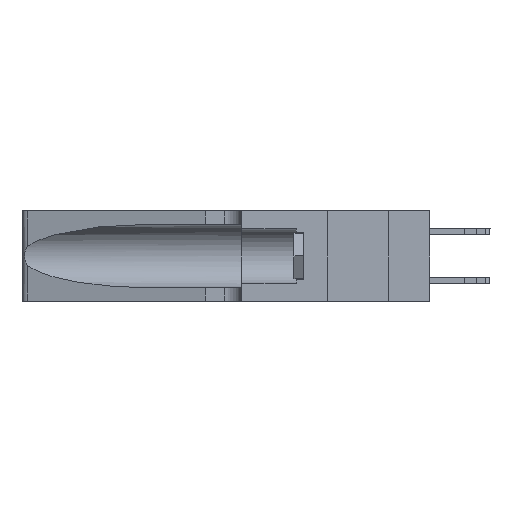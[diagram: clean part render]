
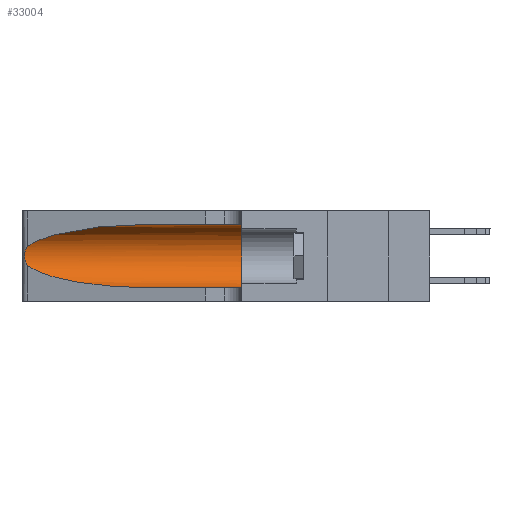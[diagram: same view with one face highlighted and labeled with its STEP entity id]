
A CAD part, left-side view. The second image highlights one B-rep face of the part: STEP entity #33004.
In plain terms, the highlighted cylindrical face has radius 3.308 mm (diameter 6.617 mm), a partial arc.
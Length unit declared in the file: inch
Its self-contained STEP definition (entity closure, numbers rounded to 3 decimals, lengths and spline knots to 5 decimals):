
#201 = CARTESIAN_POINT ( 'NONE',  ( 0.1305, 0.72297, 0.31525 ) ) ;
#750 = VERTEX_POINT ( 'NONE', #201 ) ;
#987 = VERTEX_POINT ( 'NONE', #16166 ) ;
#3765 = ORIENTED_EDGE ( 'NONE', *, *, #8868, .F. ) ;
#3880 = CARTESIAN_POINT ( 'NONE',  ( 0.2373, 1.15595, 0.08982 ) ) ;
#4283 = CARTESIAN_POINT ( 'NONE',  ( 0.1305, 0.72297, 0.05475 ) ) ;
#4322 = EDGE_CURVE ( 'NONE', #750, #6726, #26907, .T. ) ;
#4365 = CARTESIAN_POINT ( 'NONE',  ( 0.1305, 1.61858, 0.31525 ) ) ;
#5278 = ORIENTED_EDGE ( 'NONE', *, *, #11281, .T. ) ;
#5310 = CARTESIAN_POINT ( 'NONE',  ( 0.25856, 1.23593, 0.16098 ) ) ;
#6726 = VERTEX_POINT ( 'NONE', #12524 ) ;
#6749 = EDGE_CURVE ( 'NONE', #18286, #987, #23998, .T. ) ;
#8090 = CARTESIAN_POINT ( 'NONE',  ( 0.1305, 0.72297, 0.31525 ) ) ;
#8315 = VECTOR ( 'NONE', #16398, 39.37008 ) ;
#8562 = CARTESIAN_POINT ( 'NONE',  ( 0.1305, 0.35, 0.05475 ) ) ;
#8868 = EDGE_CURVE ( 'NONE', #24769, #29860, #33527, .T. ) ;
#9172 = FACE_OUTER_BOUND ( 'NONE', #18961, .T. ) ;
#9213 = LINE ( 'NONE', #10686, #8315 ) ;
#10686 = CARTESIAN_POINT ( 'NONE',  ( 0.1305, 1.61858, 0.05475 ) ) ;
#11252 = CARTESIAN_POINT ( 'NONE',  ( 0.26018, 1.23835, 0.19895 ) ) ;
#11281 = EDGE_CURVE ( 'NONE', #987, #29860, #9213, .T. ) ;
#12413 = ORIENTED_EDGE ( 'NONE', *, *, #35015, .T. ) ;
#12524 = CARTESIAN_POINT ( 'NONE',  ( 0.25487, 1.22718, 0.22369 ) ) ;
#12781 = CARTESIAN_POINT ( 'NONE',  ( 0.25487, 1.22718, 0.14631 ) ) ;
#13928 = DIRECTION ( 'NONE',  ( 0., 0., 1. ) ) ;
#14357 = CARTESIAN_POINT ( 'NONE',  ( 0.25639, 1.23184, 0.21858 ) ) ;
#15244 = CARTESIAN_POINT ( 'NONE',  ( 0.25487, 1.22718, 0.14631 ) ) ;
#15320 = AXIS2_PLACEMENT_3D ( 'NONE', #31738, #34894, #13928 ) ;
#16166 = CARTESIAN_POINT ( 'NONE',  ( 0.1305, 0.72297, 0.05475 ) ) ;
#16398 = DIRECTION ( 'NONE',  ( 0., -1., 0. ) ) ;
#17060 = CARTESIAN_POINT ( 'NONE',  ( 0.25789, 1.23486, 0.15765 ) ) ;
#18016 = CARTESIAN_POINT ( 'NONE',  ( 0.2373, 1.15595, 0.28018 ) ) ;
#18286 = VERTEX_POINT ( 'NONE', #15244 ) ;
#18961 = EDGE_LOOP ( 'NONE', ( #20723, #12413, #30042, #5278, #3765, #33374 ) ) ;
#20701 = EDGE_CURVE ( 'NONE', #750, #24769, #32829, .T. ) ;
#20723 = ORIENTED_EDGE ( 'NONE', *, *, #4322, .T. ) ;
#22903 = CARTESIAN_POINT ( 'NONE',  ( 0.25555, 1.22994, 0.2215 ) ) ;
#23026 = CARTESIAN_POINT ( 'NONE',  ( 0.25487, 1.22718, 0.22369 ) ) ;
#23134 = DIRECTION ( 'NONE',  ( 0., -1., 0. ) ) ;
#23998 =( BOUNDED_CURVE ( )  B_SPLINE_CURVE ( 3, ( #12781, #3880, #24447, #4283 ),
 .UNSPECIFIED., .F., .F. ) 
 B_SPLINE_CURVE_WITH_KNOTS ( ( 4, 4 ),
 ( 3.44316, 4.71239 ),
 .UNSPECIFIED. ) 
 CURVE ( )  GEOMETRIC_REPRESENTATION_ITEM ( )  RATIONAL_B_SPLINE_CURVE ( ( 1., 0.87, 0.87, 1. ) ) 
 REPRESENTATION_ITEM ( '' )  );
#24447 = CARTESIAN_POINT ( 'NONE',  ( 0.18966, 0.96281, 0.05475 ) ) ;
#24452 = B_SPLINE_CURVE_WITH_KNOTS ( 'NONE', 3,
 ( #23026, #22903, #14357, #25901, #34919, #11252, #32031, #28767, #37636, #5310, #17060, #28643, #26047, #37917 ),
 .UNSPECIFIED., .F., .F.,
 ( 4, 2, 2, 2, 2, 2, 4 ),
 ( 0., 0.00027, 0.00053, 0.00107, 0.0016, 0.00187, 0.00214 ),
 .UNSPECIFIED. ) ;
#24769 = VERTEX_POINT ( 'NONE', #27225 ) ;
#25901 = CARTESIAN_POINT ( 'NONE',  ( 0.25787, 1.23484, 0.2124 ) ) ;
#26047 = CARTESIAN_POINT ( 'NONE',  ( 0.25555, 1.22993, 0.14849 ) ) ;
#26164 = CARTESIAN_POINT ( 'NONE',  ( 0.1305, 1.61858, 0.185 ) ) ;
#26907 =( BOUNDED_CURVE ( )  B_SPLINE_CURVE ( 3, ( #8090, #32882, #18016, #29989 ),
 .UNSPECIFIED., .F., .T. ) 
 B_SPLINE_CURVE_WITH_KNOTS ( ( 4, 4 ),
 ( 1.5708, 2.84003 ),
 .UNSPECIFIED. ) 
 CURVE ( )  GEOMETRIC_REPRESENTATION_ITEM ( )  RATIONAL_B_SPLINE_CURVE ( ( 1., 0.87, 0.87, 1. ) ) 
 REPRESENTATION_ITEM ( '' )  );
#27225 = CARTESIAN_POINT ( 'NONE',  ( 0.1305, 0.35, 0.31525 ) ) ;
#28206 = CYLINDRICAL_SURFACE ( 'NONE', #28801, 0.13025 ) ;
#28643 = CARTESIAN_POINT ( 'NONE',  ( 0.25639, 1.23186, 0.15144 ) ) ;
#28767 = CARTESIAN_POINT ( 'NONE',  ( 0.26075, 1.23896, 0.178 ) ) ;
#28801 = AXIS2_PLACEMENT_3D ( 'NONE', #26164, #23134, #32153 ) ;
#29860 = VERTEX_POINT ( 'NONE', #8562 ) ;
#29989 = CARTESIAN_POINT ( 'NONE',  ( 0.25487, 1.22718, 0.22369 ) ) ;
#30042 = ORIENTED_EDGE ( 'NONE', *, *, #6749, .T. ) ;
#31738 = CARTESIAN_POINT ( 'NONE',  ( 0.1305, 0.35, 0.185 ) ) ;
#32031 = CARTESIAN_POINT ( 'NONE',  ( 0.26075, 1.23896, 0.19203 ) ) ;
#32153 = DIRECTION ( 'NONE',  ( 0., 0., -1. ) ) ;
#32829 = LINE ( 'NONE', #4365, #35165 ) ;
#32882 = CARTESIAN_POINT ( 'NONE',  ( 0.18966, 0.96281, 0.31525 ) ) ;
#33004 = ADVANCED_FACE ( 'NONE', ( #9172 ), #28206, .F. ) ;
#33374 = ORIENTED_EDGE ( 'NONE', *, *, #20701, .F. ) ;
#33527 = CIRCLE ( 'NONE', #15320, 0.13025 ) ;
#33810 = DIRECTION ( 'NONE',  ( 0., -1., 0. ) ) ;
#34894 = DIRECTION ( 'NONE',  ( 0., 1., 0. ) ) ;
#34919 = CARTESIAN_POINT ( 'NONE',  ( 0.25854, 1.2359, 0.20912 ) ) ;
#35015 = EDGE_CURVE ( 'NONE', #6726, #18286, #24452, .T. ) ;
#35165 = VECTOR ( 'NONE', #33810, 39.37008 ) ;
#37636 = CARTESIAN_POINT ( 'NONE',  ( 0.26017, 1.23833, 0.17102 ) ) ;
#37917 = CARTESIAN_POINT ( 'NONE',  ( 0.25487, 1.22718, 0.14631 ) ) ;
